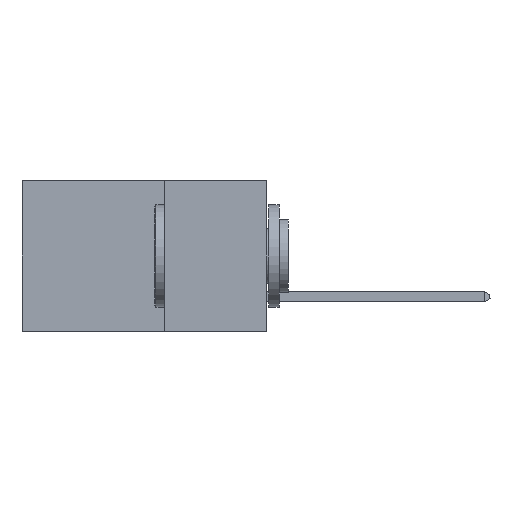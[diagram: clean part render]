
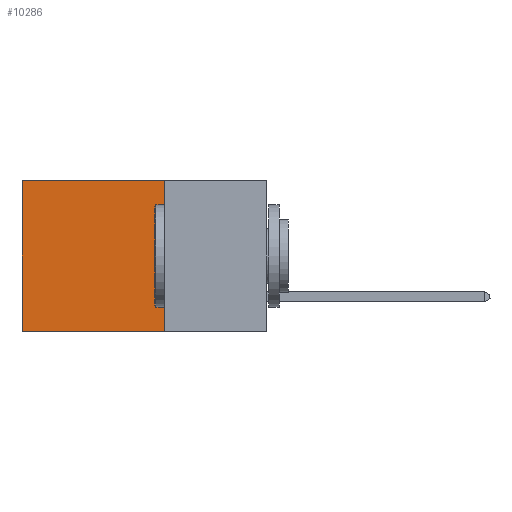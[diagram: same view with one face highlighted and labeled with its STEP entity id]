
A CAD part, left-side view. The second image highlights one B-rep face of the part: STEP entity #10286.
In plain terms, the highlighted planar face has unit normal (-1, 0, 0).
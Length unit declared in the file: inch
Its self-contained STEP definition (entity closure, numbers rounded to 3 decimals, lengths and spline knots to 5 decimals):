
#218 = VERTEX_POINT ( 'NONE', #6722 ) ;
#226 = DIRECTION ( 'NONE',  ( 0., 1., 0. ) ) ;
#347 = LINE ( 'NONE', #7510, #17987 ) ;
#842 = FACE_OUTER_BOUND ( 'NONE', #16036, .T. ) ;
#1492 = VECTOR ( 'NONE', #10921, 39.37008 ) ;
#2558 = VERTEX_POINT ( 'NONE', #10455 ) ;
#2576 = CARTESIAN_POINT ( 'NONE',  ( 0.2875, 0.25, 0. ) ) ;
#2737 = AXIS2_PLACEMENT_3D ( 'NONE', #13084, #14090, #5865 ) ;
#2769 = EDGE_CURVE ( 'NONE', #2558, #14463, #347, .T. ) ;
#3033 = VERTEX_POINT ( 'NONE', #3925 ) ;
#3075 = LINE ( 'NONE', #2576, #10062 ) ;
#3925 = CARTESIAN_POINT ( 'NONE',  ( 0.2875, 0.6, -0.37 ) ) ;
#5716 = EDGE_CURVE ( 'NONE', #2558, #218, #3075, .T. ) ;
#5865 = DIRECTION ( 'NONE',  ( 0., 0., -1. ) ) ;
#6722 = CARTESIAN_POINT ( 'NONE',  ( 0.2875, 0.6, 0. ) ) ;
#6877 = DIRECTION ( 'NONE',  ( 0., 1., 0. ) ) ;
#7072 = EDGE_CURVE ( 'NONE', #14463, #3033, #9585, .T. ) ;
#7397 = CARTESIAN_POINT ( 'NONE',  ( 0.2875, 0.25, -0.37 ) ) ;
#7510 = CARTESIAN_POINT ( 'NONE',  ( 0.2875, 0.25, 0. ) ) ;
#9168 = VECTOR ( 'NONE', #226, 39.37008 ) ;
#9585 = LINE ( 'NONE', #7397, #9168 ) ;
#9723 = ORIENTED_EDGE ( 'NONE', *, *, #2769, .F. ) ;
#9928 = PLANE ( 'NONE',  #2737 ) ;
#10062 = VECTOR ( 'NONE', #6877, 39.37008 ) ;
#10286 = ADVANCED_FACE ( 'NONE', ( #842 ), #9928, .F. ) ;
#10455 = CARTESIAN_POINT ( 'NONE',  ( 0.2875, 0.25, 0. ) ) ;
#10746 = ORIENTED_EDGE ( 'NONE', *, *, #16788, .T. ) ;
#10921 = DIRECTION ( 'NONE',  ( 0., 0., -1. ) ) ;
#11058 = ORIENTED_EDGE ( 'NONE', *, *, #5716, .T. ) ;
#12665 = LINE ( 'NONE', #17685, #1492 ) ;
#13084 = CARTESIAN_POINT ( 'NONE',  ( 0.2875, 0.25, 0. ) ) ;
#14090 = DIRECTION ( 'NONE',  ( 1., 0., 0. ) ) ;
#14463 = VERTEX_POINT ( 'NONE', #15020 ) ;
#15020 = CARTESIAN_POINT ( 'NONE',  ( 0.2875, 0.25, -0.37 ) ) ;
#15950 = DIRECTION ( 'NONE',  ( 0., 0., -1. ) ) ;
#16036 = EDGE_LOOP ( 'NONE', ( #10746, #16649, #9723, #11058 ) ) ;
#16649 = ORIENTED_EDGE ( 'NONE', *, *, #7072, .F. ) ;
#16788 = EDGE_CURVE ( 'NONE', #218, #3033, #12665, .T. ) ;
#17685 = CARTESIAN_POINT ( 'NONE',  ( 0.2875, 0.6, 0. ) ) ;
#17987 = VECTOR ( 'NONE', #15950, 39.37008 ) ;
